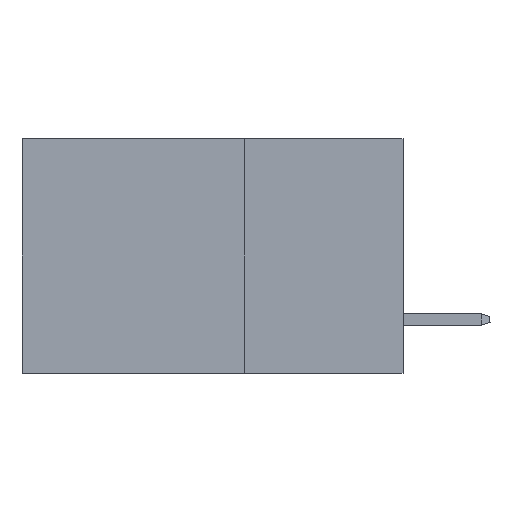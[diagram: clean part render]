
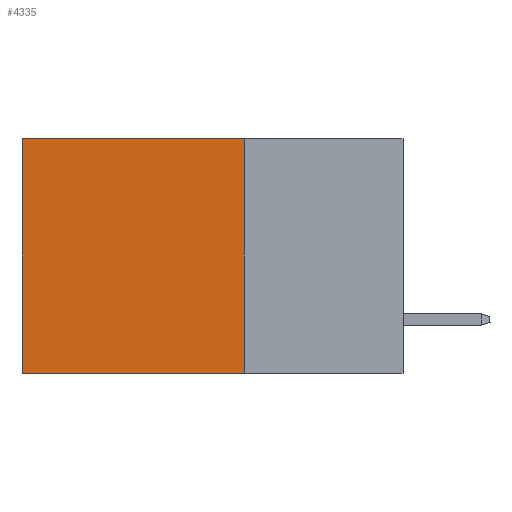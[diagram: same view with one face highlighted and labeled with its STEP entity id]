
A CAD part, left-side view. The second image highlights one B-rep face of the part: STEP entity #4335.
In plain terms, the highlighted planar face has unit normal (-1, 0, 0).
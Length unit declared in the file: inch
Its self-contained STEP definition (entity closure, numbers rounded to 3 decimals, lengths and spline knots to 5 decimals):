
#227 = DIRECTION ( 'NONE',  ( 1., 0., 0. ) ) ;
#487 = VERTEX_POINT ( 'NONE', #19177 ) ;
#1375 = EDGE_LOOP ( 'NONE', ( #13604, #18758, #27571, #37424 ) ) ;
#2533 = VECTOR ( 'NONE', #31434, 39.37008 ) ;
#2696 = CARTESIAN_POINT ( 'NONE',  ( 0.2875, 0.25, 0. ) ) ;
#3156 = CARTESIAN_POINT ( 'NONE',  ( 0.2875, 0.25, -0.37 ) ) ;
#3505 = LINE ( 'NONE', #40020, #2533 ) ;
#4137 = DIRECTION ( 'NONE',  ( 0., 0., -1. ) ) ;
#4335 = ADVANCED_FACE ( 'NONE', ( #11871 ), #25501, .F. ) ;
#6342 = LINE ( 'NONE', #2696, #15324 ) ;
#6686 = DIRECTION ( 'NONE',  ( 0., 1., 0. ) ) ;
#6944 = VERTEX_POINT ( 'NONE', #8132 ) ;
#8132 = CARTESIAN_POINT ( 'NONE',  ( 0.2875, 0.6, -0.37 ) ) ;
#9997 = VERTEX_POINT ( 'NONE', #3156 ) ;
#11643 = EDGE_CURVE ( 'NONE', #487, #9997, #3505, .T. ) ;
#11871 = FACE_OUTER_BOUND ( 'NONE', #1375, .T. ) ;
#12080 = VECTOR ( 'NONE', #4137, 39.37008 ) ;
#12446 = AXIS2_PLACEMENT_3D ( 'NONE', #31808, #227, #37329 ) ;
#12858 = DIRECTION ( 'NONE',  ( 0., 1., 0. ) ) ;
#13604 = ORIENTED_EDGE ( 'NONE', *, *, #36999, .T. ) ;
#15324 = VECTOR ( 'NONE', #12858, 39.37008 ) ;
#18758 = ORIENTED_EDGE ( 'NONE', *, *, #25859, .F. ) ;
#19119 = CARTESIAN_POINT ( 'NONE',  ( 0.2875, 0.25, -0.37 ) ) ;
#19177 = CARTESIAN_POINT ( 'NONE',  ( 0.2875, 0.25, 0. ) ) ;
#20304 = CARTESIAN_POINT ( 'NONE',  ( 0.2875, 0.6, 0. ) ) ;
#25501 = PLANE ( 'NONE',  #12446 ) ;
#25859 = EDGE_CURVE ( 'NONE', #9997, #6944, #34624, .T. ) ;
#27571 = ORIENTED_EDGE ( 'NONE', *, *, #11643, .F. ) ;
#30721 = VERTEX_POINT ( 'NONE', #20304 ) ;
#31434 = DIRECTION ( 'NONE',  ( 0., 0., -1. ) ) ;
#31808 = CARTESIAN_POINT ( 'NONE',  ( 0.2875, 0.25, 0. ) ) ;
#34624 = LINE ( 'NONE', #19119, #35217 ) ;
#35119 = CARTESIAN_POINT ( 'NONE',  ( 0.2875, 0.6, 0. ) ) ;
#35217 = VECTOR ( 'NONE', #6686, 39.37008 ) ;
#36999 = EDGE_CURVE ( 'NONE', #30721, #6944, #38781, .T. ) ;
#37253 = EDGE_CURVE ( 'NONE', #487, #30721, #6342, .T. ) ;
#37329 = DIRECTION ( 'NONE',  ( 0., 0., -1. ) ) ;
#37424 = ORIENTED_EDGE ( 'NONE', *, *, #37253, .T. ) ;
#38781 = LINE ( 'NONE', #35119, #12080 ) ;
#40020 = CARTESIAN_POINT ( 'NONE',  ( 0.2875, 0.25, 0. ) ) ;
